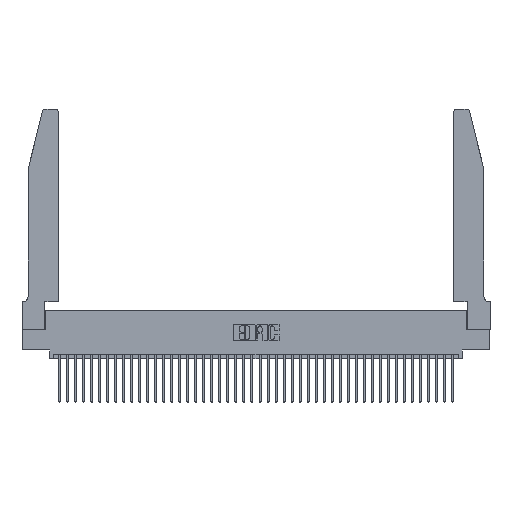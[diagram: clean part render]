
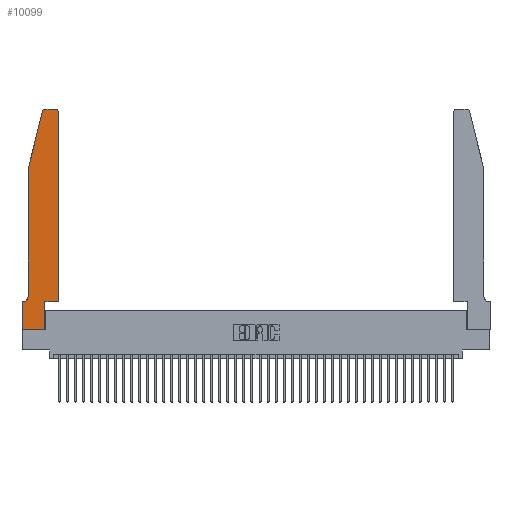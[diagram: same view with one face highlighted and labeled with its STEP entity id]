
A CAD part, top view. The second image highlights one B-rep face of the part: STEP entity #10099.
In plain terms, the highlighted planar face has unit normal (0, 0, 1).
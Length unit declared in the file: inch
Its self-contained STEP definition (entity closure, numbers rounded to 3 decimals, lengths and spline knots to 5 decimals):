
#267 = EDGE_CURVE ( 'NONE', #10214, #27747, #5401, .T. ) ;
#340 = VERTEX_POINT ( 'NONE', #2319 ) ;
#501 = VECTOR ( 'NONE', #20171, 39.37008 ) ;
#722 = ORIENTED_EDGE ( 'NONE', *, *, #8413, .T. ) ;
#784 = VECTOR ( 'NONE', #26501, 39.37008 ) ;
#1254 = CIRCLE ( 'NONE', #18225, 0.03 ) ;
#1569 = VECTOR ( 'NONE', #19618, 39.37008 ) ;
#2319 = CARTESIAN_POINT ( 'NONE',  ( 0., 0.35, 0.37 ) ) ;
#2748 = DIRECTION ( 'NONE',  ( 0., 0., 1. ) ) ;
#3189 = CARTESIAN_POINT ( 'NONE',  ( 0.4205, 2.72, 0.37 ) ) ;
#3443 = CIRCLE ( 'NONE', #11269, 0.03 ) ;
#4416 = ORIENTED_EDGE ( 'NONE', *, *, #35868, .T. ) ;
#5147 = EDGE_LOOP ( 'NONE', ( #10610, #13740, #8017, #16845, #27916, #36658, #38745, #4416, #32072, #6476, #722, #9615 ) ) ;
#5293 = DIRECTION ( 'NONE',  ( 0., 0., -1. ) ) ;
#5401 = LINE ( 'NONE', #38531, #39724 ) ;
#5514 = LINE ( 'NONE', #6899, #7582 ) ;
#5872 = EDGE_CURVE ( 'NONE', #12392, #15361, #6481, .T. ) ;
#5926 = DIRECTION ( 'NONE',  ( 1., 0., 0. ) ) ;
#6115 = DIRECTION ( 'NONE',  ( 1., 0., 0. ) ) ;
#6476 = ORIENTED_EDGE ( 'NONE', *, *, #29196, .T. ) ;
#6481 = CIRCLE ( 'NONE', #34121, 0.07 ) ;
#6517 = DIRECTION ( 'NONE',  ( 1., 0., 0. ) ) ;
#6695 = EDGE_CURVE ( 'NONE', #27144, #10214, #1254, .T. ) ;
#6899 = CARTESIAN_POINT ( 'NONE',  ( 0.0755, 2., 0.37 ) ) ;
#7582 = VECTOR ( 'NONE', #30287, 39.37008 ) ;
#8017 = ORIENTED_EDGE ( 'NONE', *, *, #13433, .T. ) ;
#8166 = VERTEX_POINT ( 'NONE', #41237 ) ;
#8336 = LINE ( 'NONE', #30164, #501 ) ;
#8405 = CARTESIAN_POINT ( 'NONE',  ( 0., 0., 0.37 ) ) ;
#8413 = EDGE_CURVE ( 'NONE', #10906, #27144, #36964, .T. ) ;
#9152 = CARTESIAN_POINT ( 'NONE',  ( 0.25487, 2.72718, 0.37 ) ) ;
#9615 = ORIENTED_EDGE ( 'NONE', *, *, #6695, .T. ) ;
#9849 = DIRECTION ( 'NONE',  ( -0.239, -0.971, 0. ) ) ;
#10099 = ADVANCED_FACE ( 'NONE', ( #33257 ), #32496, .T. ) ;
#10214 = VERTEX_POINT ( 'NONE', #19761 ) ;
#10610 = ORIENTED_EDGE ( 'NONE', *, *, #267, .T. ) ;
#10906 = VERTEX_POINT ( 'NONE', #29370 ) ;
#11269 = AXIS2_PLACEMENT_3D ( 'NONE', #22712, #2748, #26104 ) ;
#12392 = VERTEX_POINT ( 'NONE', #37115 ) ;
#13280 = VECTOR ( 'NONE', #19799, 39.37008 ) ;
#13433 = EDGE_CURVE ( 'NONE', #27204, #14557, #14138, .T. ) ;
#13740 = ORIENTED_EDGE ( 'NONE', *, *, #19272, .T. ) ;
#14138 = LINE ( 'NONE', #29747, #20925 ) ;
#14290 = LINE ( 'NONE', #36367, #13280 ) ;
#14374 = AXIS2_PLACEMENT_3D ( 'NONE', #19182, #25940, #5926 ) ;
#14557 = VERTEX_POINT ( 'NONE', #15239 ) ;
#15239 = CARTESIAN_POINT ( 'NONE',  ( 0.0755, 2., 0.37 ) ) ;
#15361 = VERTEX_POINT ( 'NONE', #42965 ) ;
#16845 = ORIENTED_EDGE ( 'NONE', *, *, #27968, .T. ) ;
#18225 = AXIS2_PLACEMENT_3D ( 'NONE', #3189, #26537, #6517 ) ;
#19182 = CARTESIAN_POINT ( 'NONE',  ( 0., 0.35, 0.37 ) ) ;
#19272 = EDGE_CURVE ( 'NONE', #27747, #27204, #3443, .T. ) ;
#19618 = DIRECTION ( 'NONE',  ( 0., 1., 0. ) ) ;
#19761 = CARTESIAN_POINT ( 'NONE',  ( 0.4205, 2.75, 0.37 ) ) ;
#19799 = DIRECTION ( 'NONE',  ( 1., 0., 0. ) ) ;
#20171 = DIRECTION ( 'NONE',  ( -1., 0., 0. ) ) ;
#20925 = VECTOR ( 'NONE', #9849, 39.37008 ) ;
#22712 = CARTESIAN_POINT ( 'NONE',  ( 0.284, 2.72, 0.37 ) ) ;
#25257 = CARTESIAN_POINT ( 'NONE',  ( 0.0055, 0.42, 0.37 ) ) ;
#25940 = DIRECTION ( 'NONE',  ( 0., 0., 1. ) ) ;
#26104 = DIRECTION ( 'NONE',  ( 1., 0., 0. ) ) ;
#26501 = DIRECTION ( 'NONE',  ( 0., 1., 0. ) ) ;
#26537 = DIRECTION ( 'NONE',  ( 0., 0., 1. ) ) ;
#27144 = VERTEX_POINT ( 'NONE', #32222 ) ;
#27204 = VERTEX_POINT ( 'NONE', #9152 ) ;
#27747 = VERTEX_POINT ( 'NONE', #29171 ) ;
#27770 = CARTESIAN_POINT ( 'NONE',  ( 0.2865, 0.35, 0.37 ) ) ;
#27903 = EDGE_CURVE ( 'NONE', #38964, #42156, #35186, .T. ) ;
#27916 = ORIENTED_EDGE ( 'NONE', *, *, #5872, .T. ) ;
#27968 = EDGE_CURVE ( 'NONE', #14557, #12392, #5514, .T. ) ;
#28445 = DIRECTION ( 'NONE',  ( 0., -1., 0. ) ) ;
#28669 = DIRECTION ( 'NONE',  ( -1., 0., 0. ) ) ;
#29171 = CARTESIAN_POINT ( 'NONE',  ( 0.284, 2.75, 0.37 ) ) ;
#29196 = EDGE_CURVE ( 'NONE', #42156, #10906, #14290, .T. ) ;
#29370 = CARTESIAN_POINT ( 'NONE',  ( 0.4505, 0.35, 0.37 ) ) ;
#29744 = CARTESIAN_POINT ( 'NONE',  ( 0.4505, 0.35, 0.37 ) ) ;
#29747 = CARTESIAN_POINT ( 'NONE',  ( 0.0755, 2., 0.37 ) ) ;
#30164 = CARTESIAN_POINT ( 'NONE',  ( 0.0755, 0.35, 0.37 ) ) ;
#30287 = DIRECTION ( 'NONE',  ( 0., -1., 0. ) ) ;
#31898 = LINE ( 'NONE', #8405, #39596 ) ;
#32071 = DIRECTION ( 'NONE',  ( -1., 0., 0. ) ) ;
#32072 = ORIENTED_EDGE ( 'NONE', *, *, #27903, .T. ) ;
#32173 = VECTOR ( 'NONE', #6115, 39.37008 ) ;
#32222 = CARTESIAN_POINT ( 'NONE',  ( 0.4505, 2.72, 0.37 ) ) ;
#32496 = PLANE ( 'NONE',  #14374 ) ;
#33257 = FACE_OUTER_BOUND ( 'NONE', #5147, .T. ) ;
#34121 = AXIS2_PLACEMENT_3D ( 'NONE', #25257, #5293, #28669 ) ;
#34987 = CARTESIAN_POINT ( 'NONE',  ( 0.2865, 0., 0.37 ) ) ;
#35186 = LINE ( 'NONE', #42938, #784 ) ;
#35868 = EDGE_CURVE ( 'NONE', #8166, #38964, #40887, .T. ) ;
#36367 = CARTESIAN_POINT ( 'NONE',  ( 0.4505, 0.35, 0.37 ) ) ;
#36658 = ORIENTED_EDGE ( 'NONE', *, *, #41249, .T. ) ;
#36964 = LINE ( 'NONE', #29744, #1569 ) ;
#37115 = CARTESIAN_POINT ( 'NONE',  ( 0.0755, 0.42, 0.37 ) ) ;
#38531 = CARTESIAN_POINT ( 'NONE',  ( 0.2605, 2.75, 0.37 ) ) ;
#38745 = ORIENTED_EDGE ( 'NONE', *, *, #40878, .T. ) ;
#38964 = VERTEX_POINT ( 'NONE', #34987 ) ;
#39281 = CARTESIAN_POINT ( 'NONE',  ( 0., 0., 0.37 ) ) ;
#39596 = VECTOR ( 'NONE', #28445, 39.37008 ) ;
#39724 = VECTOR ( 'NONE', #32071, 39.37008 ) ;
#40878 = EDGE_CURVE ( 'NONE', #340, #8166, #31898, .T. ) ;
#40887 = LINE ( 'NONE', #39281, #32173 ) ;
#41237 = CARTESIAN_POINT ( 'NONE',  ( 0., 0., 0.37 ) ) ;
#41249 = EDGE_CURVE ( 'NONE', #15361, #340, #8336, .T. ) ;
#42156 = VERTEX_POINT ( 'NONE', #27770 ) ;
#42938 = CARTESIAN_POINT ( 'NONE',  ( 0.2865, 0.35, 0.37 ) ) ;
#42965 = CARTESIAN_POINT ( 'NONE',  ( 0.0055, 0.35, 0.37 ) ) ;
